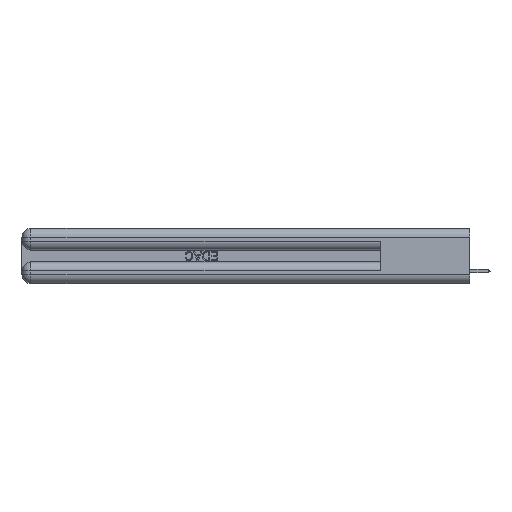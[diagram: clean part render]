
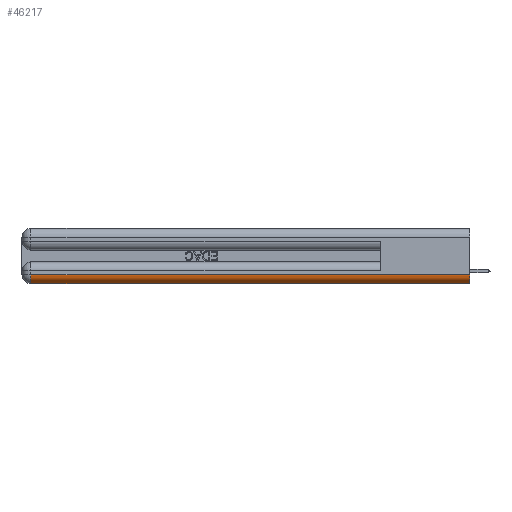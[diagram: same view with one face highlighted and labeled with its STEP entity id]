
A CAD part, left-side view. The second image highlights one B-rep face of the part: STEP entity #46217.
In plain terms, the highlighted cylindrical face has radius 1.524 mm (diameter 3.048 mm), a partial arc.
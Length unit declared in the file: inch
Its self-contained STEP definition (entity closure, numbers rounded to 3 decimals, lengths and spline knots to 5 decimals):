
#54 = VERTEX_POINT ( 'NONE', #49527 ) ;
#649 = DIRECTION ( 'NONE',  ( 0., -1., 0. ) ) ;
#945 = FACE_OUTER_BOUND ( 'NONE', #11150, .T. ) ;
#1916 = CARTESIAN_POINT ( 'NONE',  ( 0., 0., 0.06 ) ) ;
#2750 = CARTESIAN_POINT ( 'NONE',  ( 0.06, 0., 0. ) ) ;
#5107 = DIRECTION ( 'NONE',  ( 0., 1., 0. ) ) ;
#11150 = EDGE_LOOP ( 'NONE', ( #34331, #14949, #13837, #30627 ) ) ;
#13837 = ORIENTED_EDGE ( 'NONE', *, *, #23634, .F. ) ;
#14949 = ORIENTED_EDGE ( 'NONE', *, *, #49422, .F. ) ;
#21223 = VECTOR ( 'NONE', #5107, 39.37008 ) ;
#21407 = AXIS2_PLACEMENT_3D ( 'NONE', #38329, #49621, #23216 ) ;
#21868 = CIRCLE ( 'NONE', #33298, 0.06 ) ;
#23216 = DIRECTION ( 'NONE',  ( 0., 0., 1. ) ) ;
#23634 = EDGE_CURVE ( 'NONE', #54, #44858, #46129, .T. ) ;
#25547 = VERTEX_POINT ( 'NONE', #1916 ) ;
#26693 = DIRECTION ( 'NONE',  ( 0., 0., 1. ) ) ;
#27275 = DIRECTION ( 'NONE',  ( 0., 0., 1. ) ) ;
#29612 = CARTESIAN_POINT ( 'NONE',  ( 0., 2.94, 0.06 ) ) ;
#30627 = ORIENTED_EDGE ( 'NONE', *, *, #45177, .F. ) ;
#33298 = AXIS2_PLACEMENT_3D ( 'NONE', #49684, #34413, #26693 ) ;
#33885 = LINE ( 'NONE', #36185, #21223 ) ;
#34331 = ORIENTED_EDGE ( 'NONE', *, *, #44987, .F. ) ;
#34413 = DIRECTION ( 'NONE',  ( 0., -1., 0. ) ) ;
#35160 = CARTESIAN_POINT ( 'NONE',  ( 0., 0., 0.06 ) ) ;
#36185 = CARTESIAN_POINT ( 'NONE',  ( 0.06, 3., 0. ) ) ;
#37102 = CYLINDRICAL_SURFACE ( 'NONE', #48058, 0.06 ) ;
#38052 = LINE ( 'NONE', #35160, #48260 ) ;
#38329 = CARTESIAN_POINT ( 'NONE',  ( 0.06, 2.94, 0.06 ) ) ;
#41248 = DIRECTION ( 'NONE',  ( 0., 1., 0. ) ) ;
#44858 = VERTEX_POINT ( 'NONE', #29612 ) ;
#44987 = EDGE_CURVE ( 'NONE', #25547, #46674, #21868, .T. ) ;
#45177 = EDGE_CURVE ( 'NONE', #46674, #54, #33885, .T. ) ;
#46129 = CIRCLE ( 'NONE', #21407, 0.06 ) ;
#46217 = ADVANCED_FACE ( 'NONE', ( #945 ), #37102, .T. ) ;
#46674 = VERTEX_POINT ( 'NONE', #2750 ) ;
#48058 = AXIS2_PLACEMENT_3D ( 'NONE', #49648, #41248, #27275 ) ;
#48260 = VECTOR ( 'NONE', #649, 39.37008 ) ;
#49422 = EDGE_CURVE ( 'NONE', #44858, #25547, #38052, .T. ) ;
#49527 = CARTESIAN_POINT ( 'NONE',  ( 0.06, 2.94, 0. ) ) ;
#49621 = DIRECTION ( 'NONE',  ( 0., 1., 0. ) ) ;
#49648 = CARTESIAN_POINT ( 'NONE',  ( 0.06, 0., 0.06 ) ) ;
#49684 = CARTESIAN_POINT ( 'NONE',  ( 0.06, 0., 0.06 ) ) ;
